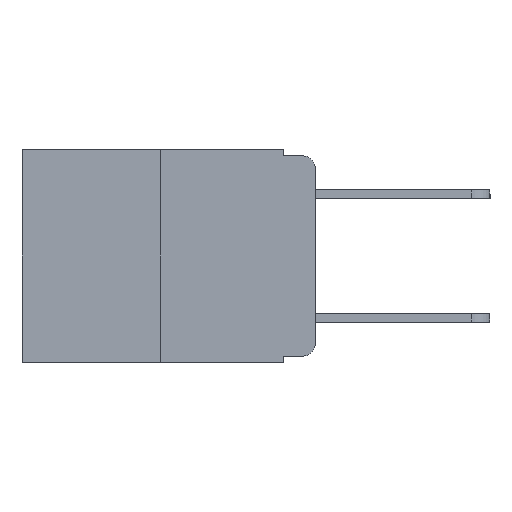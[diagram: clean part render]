
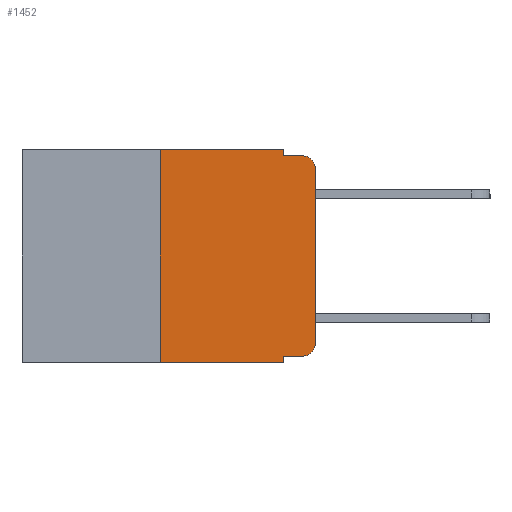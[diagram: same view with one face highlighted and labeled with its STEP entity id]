
A CAD part, left-side view. The second image highlights one B-rep face of the part: STEP entity #1452.
In plain terms, the highlighted planar face has unit normal (-1, 0, 0).
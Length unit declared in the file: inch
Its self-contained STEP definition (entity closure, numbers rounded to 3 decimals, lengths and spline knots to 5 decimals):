
#612 = ORIENTED_EDGE ( 'NONE', *, *, #9261, .F. ) ;
#646 = LINE ( 'NONE', #16571, #14742 ) ;
#1452 = ADVANCED_FACE ( 'NONE', ( #16138 ), #7916, .F. ) ;
#1596 = VERTEX_POINT ( 'NONE', #5423 ) ;
#2049 = VERTEX_POINT ( 'NONE', #4636 ) ;
#2126 = CARTESIAN_POINT ( 'NONE',  ( 0., 0.25, -0.343 ) ) ;
#2206 = CARTESIAN_POINT ( 'NONE',  ( 0., 0.02, -0.01 ) ) ;
#3637 = CARTESIAN_POINT ( 'NONE',  ( 0., 0.02, -0.03 ) ) ;
#3714 = ORIENTED_EDGE ( 'NONE', *, *, #9358, .T. ) ;
#3771 = CARTESIAN_POINT ( 'NONE',  ( 0., 0.25, 0. ) ) ;
#4080 = CARTESIAN_POINT ( 'NONE',  ( 0., 0.02, -0.313 ) ) ;
#4338 = VERTEX_POINT ( 'NONE', #12189 ) ;
#4628 = LINE ( 'NONE', #7933, #11293 ) ;
#4636 = CARTESIAN_POINT ( 'NONE',  ( 0., 0.02, -0.333 ) ) ;
#4985 = AXIS2_PLACEMENT_3D ( 'NONE', #9065, #14632, #7762 ) ;
#5042 = LINE ( 'NONE', #3771, #15099 ) ;
#5096 = DIRECTION ( 'NONE',  ( 0., 0., -1. ) ) ;
#5411 = AXIS2_PLACEMENT_3D ( 'NONE', #4080, #13446, #5489 ) ;
#5423 = CARTESIAN_POINT ( 'NONE',  ( 0., 0.051, -0.333 ) ) ;
#5489 = DIRECTION ( 'NONE',  ( 0., 0., -1. ) ) ;
#5634 = LINE ( 'NONE', #11788, #12319 ) ;
#5825 = VERTEX_POINT ( 'NONE', #2126 ) ;
#6331 = EDGE_CURVE ( 'NONE', #10420, #10372, #646, .T. ) ;
#6540 = CIRCLE ( 'NONE', #5411, 0.02 ) ;
#6773 = DIRECTION ( 'NONE',  ( 0., -1., 0. ) ) ;
#6974 = ORIENTED_EDGE ( 'NONE', *, *, #9241, .T. ) ;
#6985 = VECTOR ( 'NONE', #6773, 39.37008 ) ;
#7276 = EDGE_CURVE ( 'NONE', #5825, #15088, #9375, .T. ) ;
#7725 = CARTESIAN_POINT ( 'NONE',  ( 0., 0., 0. ) ) ;
#7762 = DIRECTION ( 'NONE',  ( 0., 0., -1. ) ) ;
#7778 = CARTESIAN_POINT ( 'NONE',  ( 0., 0.051, -0.01 ) ) ;
#7916 = PLANE ( 'NONE',  #4985 ) ;
#7933 = CARTESIAN_POINT ( 'NONE',  ( 0., 0.051, 0. ) ) ;
#8043 = CARTESIAN_POINT ( 'NONE',  ( 0., 0.051, -0.333 ) ) ;
#8995 = AXIS2_PLACEMENT_3D ( 'NONE', #3637, #13022, #5096 ) ;
#9064 = DIRECTION ( 'NONE',  ( 0., 0., 1. ) ) ;
#9065 = CARTESIAN_POINT ( 'NONE',  ( 0., 0.473, 0. ) ) ;
#9121 = DIRECTION ( 'NONE',  ( 0., -1., 0. ) ) ;
#9193 = VECTOR ( 'NONE', #9121, 39.37008 ) ;
#9239 = EDGE_CURVE ( 'NONE', #9610, #4338, #13935, .T. ) ;
#9241 = EDGE_CURVE ( 'NONE', #4338, #10022, #13083, .T. ) ;
#9261 = EDGE_CURVE ( 'NONE', #10157, #10022, #13536, .T. ) ;
#9264 = EDGE_CURVE ( 'NONE', #10372, #10157, #5634, .T. ) ;
#9291 = EDGE_CURVE ( 'NONE', #5825, #10420, #5042, .T. ) ;
#9315 = EDGE_CURVE ( 'NONE', #1596, #15088, #4628, .T. ) ;
#9338 = EDGE_CURVE ( 'NONE', #1596, #2049, #14361, .T. ) ;
#9358 = EDGE_CURVE ( 'NONE', #2049, #9610, #6540, .T. ) ;
#9375 = LINE ( 'NONE', #12777, #12883 ) ;
#9610 = VERTEX_POINT ( 'NONE', #15629 ) ;
#9612 = VECTOR ( 'NONE', #9064, 39.37008 ) ;
#10022 = VERTEX_POINT ( 'NONE', #2206 ) ;
#10157 = VERTEX_POINT ( 'NONE', #10671 ) ;
#10372 = VERTEX_POINT ( 'NONE', #14790 ) ;
#10420 = VERTEX_POINT ( 'NONE', #13585 ) ;
#10671 = CARTESIAN_POINT ( 'NONE',  ( 0., 0.051, -0.01 ) ) ;
#11187 = EDGE_LOOP ( 'NONE', ( #12121, #6974, #612, #15190, #13796, #14300, #15914, #15685, #15632, #3714 ) ) ;
#11293 = VECTOR ( 'NONE', #15700, 39.37008 ) ;
#11468 = DIRECTION ( 'NONE',  ( 0., -1., 0. ) ) ;
#11788 = CARTESIAN_POINT ( 'NONE',  ( 0., 0.051, 0. ) ) ;
#12121 = ORIENTED_EDGE ( 'NONE', *, *, #9239, .T. ) ;
#12189 = CARTESIAN_POINT ( 'NONE',  ( 0., 0., -0.03 ) ) ;
#12319 = VECTOR ( 'NONE', #13064, 39.37008 ) ;
#12777 = CARTESIAN_POINT ( 'NONE',  ( 0., 0.473, -0.343 ) ) ;
#12883 = VECTOR ( 'NONE', #11468, 39.37008 ) ;
#13022 = DIRECTION ( 'NONE',  ( -1., 0., 0. ) ) ;
#13064 = DIRECTION ( 'NONE',  ( 0., 0., -1. ) ) ;
#13083 = CIRCLE ( 'NONE', #8995, 0.02 ) ;
#13128 = DIRECTION ( 'NONE',  ( 0., 0., 1. ) ) ;
#13446 = DIRECTION ( 'NONE',  ( -1., 0., 0. ) ) ;
#13536 = LINE ( 'NONE', #7778, #9193 ) ;
#13585 = CARTESIAN_POINT ( 'NONE',  ( 0., 0.25, 0. ) ) ;
#13796 = ORIENTED_EDGE ( 'NONE', *, *, #6331, .F. ) ;
#13935 = LINE ( 'NONE', #7725, #9612 ) ;
#14240 = DIRECTION ( 'NONE',  ( 0., -1., 0. ) ) ;
#14300 = ORIENTED_EDGE ( 'NONE', *, *, #9291, .F. ) ;
#14361 = LINE ( 'NONE', #8043, #6985 ) ;
#14632 = DIRECTION ( 'NONE',  ( 1., 0., 0. ) ) ;
#14742 = VECTOR ( 'NONE', #14240, 39.37008 ) ;
#14790 = CARTESIAN_POINT ( 'NONE',  ( 0., 0.051, 0. ) ) ;
#15088 = VERTEX_POINT ( 'NONE', #16200 ) ;
#15099 = VECTOR ( 'NONE', #13128, 39.37008 ) ;
#15190 = ORIENTED_EDGE ( 'NONE', *, *, #9264, .F. ) ;
#15629 = CARTESIAN_POINT ( 'NONE',  ( 0., 0., -0.313 ) ) ;
#15632 = ORIENTED_EDGE ( 'NONE', *, *, #9338, .T. ) ;
#15685 = ORIENTED_EDGE ( 'NONE', *, *, #9315, .F. ) ;
#15700 = DIRECTION ( 'NONE',  ( 0., 0., -1. ) ) ;
#15914 = ORIENTED_EDGE ( 'NONE', *, *, #7276, .T. ) ;
#16138 = FACE_OUTER_BOUND ( 'NONE', #11187, .T. ) ;
#16200 = CARTESIAN_POINT ( 'NONE',  ( 0., 0.051, -0.343 ) ) ;
#16571 = CARTESIAN_POINT ( 'NONE',  ( 0., 0.473, 0. ) ) ;
